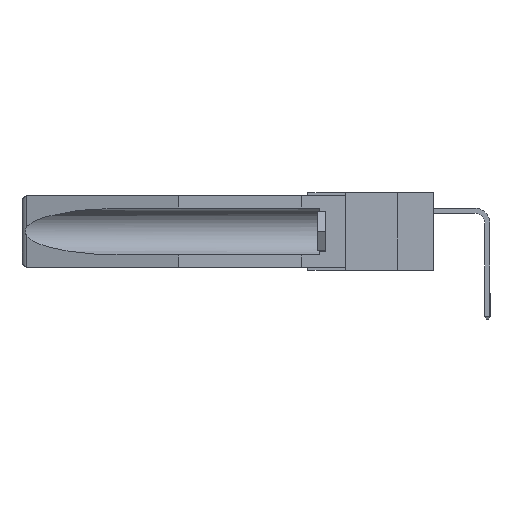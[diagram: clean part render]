
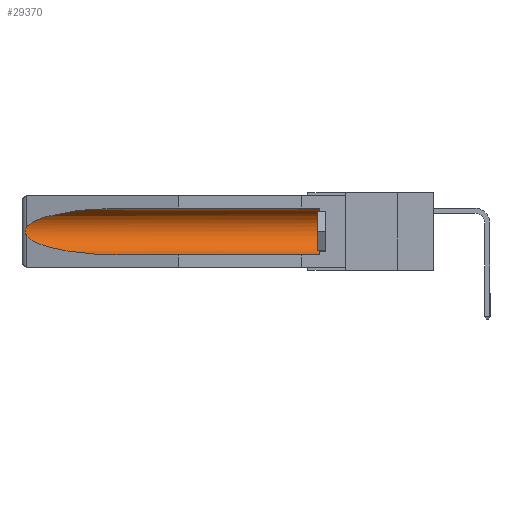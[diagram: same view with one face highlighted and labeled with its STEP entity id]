
A CAD part, left-side view. The second image highlights one B-rep face of the part: STEP entity #29370.
In plain terms, the highlighted cylindrical face has radius 2.857 mm (diameter 5.715 mm), a partial arc.
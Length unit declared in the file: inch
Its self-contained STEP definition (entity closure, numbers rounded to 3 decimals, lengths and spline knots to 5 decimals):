
#201 = CARTESIAN_POINT ( 'NONE',  ( 0.26597, 1.5296, -0.19026 ) ) ;
#1197 = EDGE_CURVE ( 'NONE', #5485, #16242, #21056, .T. ) ;
#1344 = CARTESIAN_POINT ( 'NONE',  ( 0.155, 1.07973, -0.059 ) ) ;
#1860 = VERTEX_POINT ( 'NONE', #8024 ) ;
#2277 = FACE_OUTER_BOUND ( 'NONE', #5322, .T. ) ;
#2632 = CARTESIAN_POINT ( 'NONE',  ( 0.2675, 1.53308, -0.17534 ) ) ;
#3427 = CARTESIAN_POINT ( 'NONE',  ( 0.25451, 1.48313, -0.09465 ) ) ;
#3533 = VECTOR ( 'NONE', #17474, 39.37008 ) ;
#5253 = CARTESIAN_POINT ( 'NONE',  ( 0.2673, 1.5327, -0.16383 ) ) ;
#5322 = EDGE_LOOP ( 'NONE', ( #18120, #31471, #8321, #10645, #19769, #31048 ) ) ;
#5485 = VERTEX_POINT ( 'NONE', #16248 ) ;
#5625 = CARTESIAN_POINT ( 'NONE',  ( 0.25451, 1.48313, -0.24835 ) ) ;
#5856 = CARTESIAN_POINT ( 'NONE',  ( 0.21114, 1.30732, -0.059 ) ) ;
#6171 = EDGE_CURVE ( 'NONE', #7022, #25770, #10624, .T. ) ;
#7022 = VERTEX_POINT ( 'NONE', #22154 ) ;
#8024 = CARTESIAN_POINT ( 'NONE',  ( 0.155, 0.126, -0.059 ) ) ;
#8062 = CARTESIAN_POINT ( 'NONE',  ( 0.155, 1.07973, -0.284 ) ) ;
#8321 = ORIENTED_EDGE ( 'NONE', *, *, #19930, .T. ) ;
#8498 = CARTESIAN_POINT ( 'NONE',  ( 0.21114, 1.30732, -0.284 ) ) ;
#8815 = LINE ( 'NONE', #15252, #10816 ) ;
#9126 = EDGE_CURVE ( 'NONE', #1860, #5485, #8815, .T. ) ;
#9344 = DIRECTION ( 'NONE',  ( 0., -1., 0. ) ) ;
#9749 = CARTESIAN_POINT ( 'NONE',  ( 0.155, 1.07973, -0.284 ) ) ;
#10125 = CARTESIAN_POINT ( 'NONE',  ( 0.26537, 1.52718, -0.19328 ) ) ;
#10624 = LINE ( 'NONE', #12395, #3533 ) ;
#10645 = ORIENTED_EDGE ( 'NONE', *, *, #6171, .F. ) ;
#10689 = VERTEX_POINT ( 'NONE', #26210 ) ;
#10816 = VECTOR ( 'NONE', #30460, 39.37008 ) ;
#11141 = CARTESIAN_POINT ( 'NONE',  ( 0.26537, 1.52718, -0.14972 ) ) ;
#11513 = CIRCLE ( 'NONE', #22630, 0.1125 ) ;
#12395 = CARTESIAN_POINT ( 'NONE',  ( 0.155, -0.30754, -0.284 ) ) ;
#12789 = B_SPLINE_CURVE_WITH_KNOTS ( 'NONE', 3,
 ( #19920, #27509, #17722, #5253, #15417, #2632, #22757, #30285, #201, #10125 ),
 .UNSPECIFIED., .F., .F.,
 ( 4, 2, 2, 2, 4 ),
 ( 0., 0.00029, 0.00058, 0.00087, 0.00117 ),
 .UNSPECIFIED. ) ;
#15252 = CARTESIAN_POINT ( 'NONE',  ( 0.155, -0.30754, -0.059 ) ) ;
#15417 = CARTESIAN_POINT ( 'NONE',  ( 0.2675, 1.53308, -0.16763 ) ) ;
#16242 = VERTEX_POINT ( 'NONE', #28540 ) ;
#16248 = CARTESIAN_POINT ( 'NONE',  ( 0.155, 1.07973, -0.059 ) ) ;
#16452 = EDGE_CURVE ( 'NONE', #7022, #1860, #11513, .T. ) ;
#16846 = CARTESIAN_POINT ( 'NONE',  ( 0.155, 0.126, -0.1715 ) ) ;
#17272 = DIRECTION ( 'NONE',  ( 0., 0., 1. ) ) ;
#17474 = DIRECTION ( 'NONE',  ( 0., 1., 0. ) ) ;
#17722 = CARTESIAN_POINT ( 'NONE',  ( 0.26654, 1.53092, -0.15636 ) ) ;
#18120 = ORIENTED_EDGE ( 'NONE', *, *, #1197, .T. ) ;
#18276 = AXIS2_PLACEMENT_3D ( 'NONE', #32478, #27067, #24634 ) ;
#19769 = ORIENTED_EDGE ( 'NONE', *, *, #16452, .T. ) ;
#19920 = CARTESIAN_POINT ( 'NONE',  ( 0.26537, 1.52718, -0.14972 ) ) ;
#19930 = EDGE_CURVE ( 'NONE', #10689, #25770, #32377, .T. ) ;
#21056 =( BOUNDED_CURVE ( )  B_SPLINE_CURVE ( 3, ( #1344, #5856, #3427, #11141 ),
 .UNSPECIFIED., .F., .F. ) 
 B_SPLINE_CURVE_WITH_KNOTS ( ( 4, 4 ),
 ( 4.71239, 6.08839 ),
 .UNSPECIFIED. ) 
 CURVE ( )  GEOMETRIC_REPRESENTATION_ITEM ( )  RATIONAL_B_SPLINE_CURVE ( ( 1., 0.848, 0.848, 1. ) ) 
 REPRESENTATION_ITEM ( '' )  );
#22154 = CARTESIAN_POINT ( 'NONE',  ( 0.155, 0.126, -0.284 ) ) ;
#22630 = AXIS2_PLACEMENT_3D ( 'NONE', #16846, #9344, #17272 ) ;
#22757 = CARTESIAN_POINT ( 'NONE',  ( 0.2673, 1.53269, -0.17917 ) ) ;
#24634 = DIRECTION ( 'NONE',  ( 0., 0., 1. ) ) ;
#25183 = EDGE_CURVE ( 'NONE', #16242, #10689, #12789, .T. ) ;
#25770 = VERTEX_POINT ( 'NONE', #9749 ) ;
#26210 = CARTESIAN_POINT ( 'NONE',  ( 0.26537, 1.52718, -0.19328 ) ) ;
#27067 = DIRECTION ( 'NONE',  ( 0., 1., 0. ) ) ;
#27074 = CYLINDRICAL_SURFACE ( 'NONE', #18276, 0.1125 ) ;
#27509 = CARTESIAN_POINT ( 'NONE',  ( 0.26597, 1.52961, -0.15275 ) ) ;
#28540 = CARTESIAN_POINT ( 'NONE',  ( 0.26537, 1.52718, -0.14972 ) ) ;
#29370 = ADVANCED_FACE ( 'NONE', ( #2277 ), #27074, .F. ) ;
#30285 = CARTESIAN_POINT ( 'NONE',  ( 0.26655, 1.53094, -0.18657 ) ) ;
#30460 = DIRECTION ( 'NONE',  ( 0., 1., 0. ) ) ;
#30859 = CARTESIAN_POINT ( 'NONE',  ( 0.26537, 1.52718, -0.19328 ) ) ;
#31048 = ORIENTED_EDGE ( 'NONE', *, *, #9126, .T. ) ;
#31471 = ORIENTED_EDGE ( 'NONE', *, *, #25183, .T. ) ;
#32377 =( BOUNDED_CURVE ( )  B_SPLINE_CURVE ( 3, ( #30859, #5625, #8498, #8062 ),
 .UNSPECIFIED., .F., .F. ) 
 B_SPLINE_CURVE_WITH_KNOTS ( ( 4, 4 ),
 ( 0.1948, 1.5708 ),
 .UNSPECIFIED. ) 
 CURVE ( )  GEOMETRIC_REPRESENTATION_ITEM ( )  RATIONAL_B_SPLINE_CURVE ( ( 1., 0.848, 0.848, 1. ) ) 
 REPRESENTATION_ITEM ( '' )  );
#32478 = CARTESIAN_POINT ( 'NONE',  ( 0.155, -0.30754, -0.1715 ) ) ;
